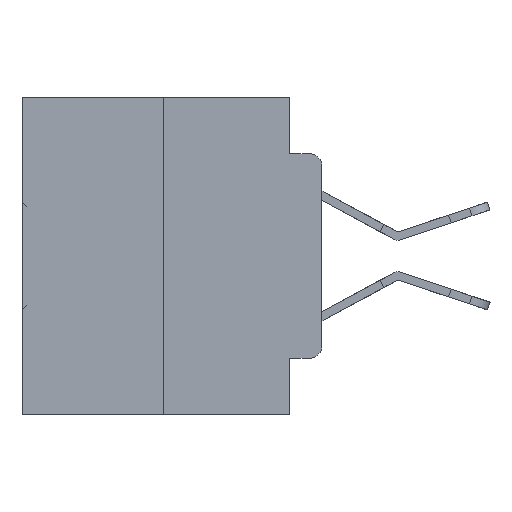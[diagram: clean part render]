
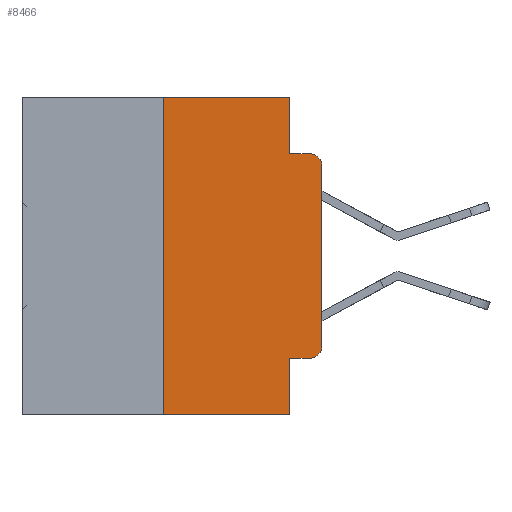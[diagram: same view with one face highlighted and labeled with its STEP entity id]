
A CAD part, left-side view. The second image highlights one B-rep face of the part: STEP entity #8466.
In plain terms, the highlighted planar face has unit normal (-1, 0, 0).
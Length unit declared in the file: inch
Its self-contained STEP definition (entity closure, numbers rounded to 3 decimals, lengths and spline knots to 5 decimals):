
#400 = DIRECTION ( 'NONE',  ( 0., 0., -1. ) ) ;
#446 = VERTEX_POINT ( 'NONE', #11063 ) ;
#519 = ORIENTED_EDGE ( 'NONE', *, *, #33578, .F. ) ;
#752 = CARTESIAN_POINT ( 'NONE',  ( 0., 0.051, -0.4115 ) ) ;
#1051 = LINE ( 'NONE', #34417, #31511 ) ;
#1305 = LINE ( 'NONE', #752, #31566 ) ;
#1463 = CARTESIAN_POINT ( 'NONE',  ( 0., 0.02, -0.1085 ) ) ;
#1626 = LINE ( 'NONE', #26955, #18547 ) ;
#3053 = DIRECTION ( 'NONE',  ( 0., -1., 0. ) ) ;
#3471 = EDGE_CURVE ( 'NONE', #8997, #32523, #17909, .T. ) ;
#5390 = DIRECTION ( 'NONE',  ( 0., 0., 1. ) ) ;
#6261 = ORIENTED_EDGE ( 'NONE', *, *, #10699, .T. ) ;
#6299 = CARTESIAN_POINT ( 'NONE',  ( 0., 0.02, -0.0885 ) ) ;
#6378 = DIRECTION ( 'NONE',  ( 0., -1., 0. ) ) ;
#7658 = AXIS2_PLACEMENT_3D ( 'NONE', #1463, #34833, #28830 ) ;
#7780 = LINE ( 'NONE', #24371, #8762 ) ;
#8466 = ADVANCED_FACE ( 'NONE', ( #28554 ), #33842, .F. ) ;
#8702 = LINE ( 'NONE', #22916, #14536 ) ;
#8762 = VECTOR ( 'NONE', #5390, 39.37008 ) ;
#8912 = CARTESIAN_POINT ( 'NONE',  ( 0., 0.051, 0. ) ) ;
#8997 = VERTEX_POINT ( 'NONE', #20270 ) ;
#9026 = DIRECTION ( 'NONE',  ( 0., 0., -1. ) ) ;
#9868 = ORIENTED_EDGE ( 'NONE', *, *, #26708, .T. ) ;
#10053 = CARTESIAN_POINT ( 'NONE',  ( 0., 0., -0.1085 ) ) ;
#10589 = VECTOR ( 'NONE', #25866, 39.37008 ) ;
#10699 = EDGE_CURVE ( 'NONE', #11332, #22545, #17550, .T. ) ;
#10780 = ORIENTED_EDGE ( 'NONE', *, *, #3471, .T. ) ;
#11063 = CARTESIAN_POINT ( 'NONE',  ( 0., 0.051, -0.5 ) ) ;
#11332 = VERTEX_POINT ( 'NONE', #10053 ) ;
#11396 = ORIENTED_EDGE ( 'NONE', *, *, #30200, .T. ) ;
#11878 = ORIENTED_EDGE ( 'NONE', *, *, #27693, .T. ) ;
#13648 = CARTESIAN_POINT ( 'NONE',  ( 0., 0.25, 0. ) ) ;
#14536 = VECTOR ( 'NONE', #3053, 39.37008 ) ;
#15608 = VERTEX_POINT ( 'NONE', #13648 ) ;
#15878 = CARTESIAN_POINT ( 'NONE',  ( 0., 0.051, -0.0885 ) ) ;
#17550 = CIRCLE ( 'NONE', #7658, 0.02 ) ;
#17844 = CARTESIAN_POINT ( 'NONE',  ( 0., 0.051, -0.0885 ) ) ;
#17909 = CIRCLE ( 'NONE', #19634, 0.02 ) ;
#18547 = VECTOR ( 'NONE', #26592, 39.37008 ) ;
#18905 = CARTESIAN_POINT ( 'NONE',  ( 0., 0.25, 0. ) ) ;
#19240 = CARTESIAN_POINT ( 'NONE',  ( 0., 0.473, -0.5 ) ) ;
#19634 = AXIS2_PLACEMENT_3D ( 'NONE', #35966, #24672, #400 ) ;
#19790 = EDGE_CURVE ( 'NONE', #26275, #15608, #24389, .T. ) ;
#20005 = CARTESIAN_POINT ( 'NONE',  ( 0., 0.051, -0.4115 ) ) ;
#20270 = CARTESIAN_POINT ( 'NONE',  ( 0., 0.02, -0.4115 ) ) ;
#20288 = CARTESIAN_POINT ( 'NONE',  ( 0., 0., -0.3915 ) ) ;
#20601 = VERTEX_POINT ( 'NONE', #15878 ) ;
#21005 = EDGE_LOOP ( 'NONE', ( #9868, #6261, #24227, #30397, #31573, #34538, #11396, #519, #11878, #10780 ) ) ;
#22545 = VERTEX_POINT ( 'NONE', #6299 ) ;
#22916 = CARTESIAN_POINT ( 'NONE',  ( 0., 0.473, 0. ) ) ;
#23476 = DIRECTION ( 'NONE',  ( 0., 0., -1. ) ) ;
#23986 = EDGE_CURVE ( 'NONE', #15608, #32089, #8702, .T. ) ;
#24028 = DIRECTION ( 'NONE',  ( 0., 0., 1. ) ) ;
#24227 = ORIENTED_EDGE ( 'NONE', *, *, #28198, .F. ) ;
#24250 = VECTOR ( 'NONE', #27462, 39.37008 ) ;
#24371 = CARTESIAN_POINT ( 'NONE',  ( 0., 0., 0. ) ) ;
#24389 = LINE ( 'NONE', #18905, #31772 ) ;
#24672 = DIRECTION ( 'NONE',  ( -1., 0., 0. ) ) ;
#25272 = DIRECTION ( 'NONE',  ( 1., 0., 0. ) ) ;
#25866 = DIRECTION ( 'NONE',  ( 0., -1., 0. ) ) ;
#26275 = VERTEX_POINT ( 'NONE', #32144 ) ;
#26592 = DIRECTION ( 'NONE',  ( 0., 0., -1. ) ) ;
#26611 = EDGE_CURVE ( 'NONE', #32089, #20601, #1051, .T. ) ;
#26708 = EDGE_CURVE ( 'NONE', #32523, #11332, #7780, .T. ) ;
#26955 = CARTESIAN_POINT ( 'NONE',  ( 0., 0.051, 0. ) ) ;
#27462 = DIRECTION ( 'NONE',  ( 0., -1., 0. ) ) ;
#27693 = EDGE_CURVE ( 'NONE', #29855, #8997, #1305, .T. ) ;
#28017 = CARTESIAN_POINT ( 'NONE',  ( 0., 0.473, 0. ) ) ;
#28198 = EDGE_CURVE ( 'NONE', #20601, #22545, #28623, .T. ) ;
#28487 = AXIS2_PLACEMENT_3D ( 'NONE', #28017, #25272, #9026 ) ;
#28554 = FACE_OUTER_BOUND ( 'NONE', #21005, .T. ) ;
#28623 = LINE ( 'NONE', #17844, #10589 ) ;
#28830 = DIRECTION ( 'NONE',  ( 0., 0., -1. ) ) ;
#29855 = VERTEX_POINT ( 'NONE', #20005 ) ;
#30200 = EDGE_CURVE ( 'NONE', #26275, #446, #33467, .T. ) ;
#30397 = ORIENTED_EDGE ( 'NONE', *, *, #26611, .F. ) ;
#31511 = VECTOR ( 'NONE', #23476, 39.37008 ) ;
#31566 = VECTOR ( 'NONE', #6378, 39.37008 ) ;
#31573 = ORIENTED_EDGE ( 'NONE', *, *, #23986, .F. ) ;
#31772 = VECTOR ( 'NONE', #24028, 39.37008 ) ;
#32089 = VERTEX_POINT ( 'NONE', #8912 ) ;
#32144 = CARTESIAN_POINT ( 'NONE',  ( 0., 0.25, -0.5 ) ) ;
#32523 = VERTEX_POINT ( 'NONE', #20288 ) ;
#33467 = LINE ( 'NONE', #19240, #24250 ) ;
#33578 = EDGE_CURVE ( 'NONE', #29855, #446, #1626, .T. ) ;
#33842 = PLANE ( 'NONE',  #28487 ) ;
#34417 = CARTESIAN_POINT ( 'NONE',  ( 0., 0.051, 0. ) ) ;
#34538 = ORIENTED_EDGE ( 'NONE', *, *, #19790, .F. ) ;
#34833 = DIRECTION ( 'NONE',  ( -1., 0., 0. ) ) ;
#35966 = CARTESIAN_POINT ( 'NONE',  ( 0., 0.02, -0.3915 ) ) ;
